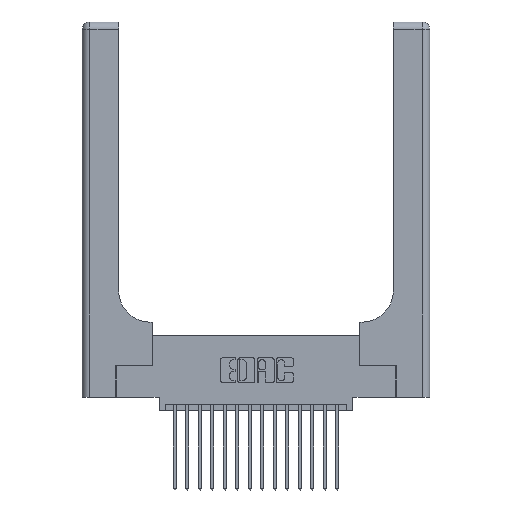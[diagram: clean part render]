
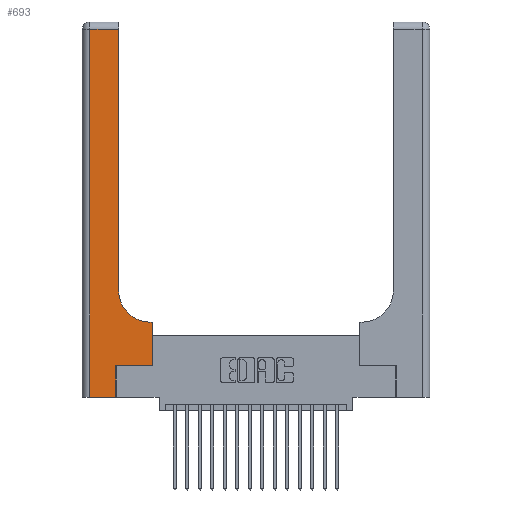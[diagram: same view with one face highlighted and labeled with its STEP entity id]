
A CAD part, top view. The second image highlights one B-rep face of the part: STEP entity #693.
In plain terms, the highlighted planar face has unit normal (0, 0, 1).
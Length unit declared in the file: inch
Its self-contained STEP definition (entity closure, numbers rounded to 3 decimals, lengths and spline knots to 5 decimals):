
#476 = PLANE ( 'NONE',  #8437 ) ;
#693 = ADVANCED_FACE ( 'NONE', ( #14383 ), #476, .F. ) ;
#715 = CARTESIAN_POINT ( 'NONE',  ( 0.5585, 0.25, 0.37 ) ) ;
#745 = CARTESIAN_POINT ( 'NONE',  ( 0.06, 2.94, 0.37 ) ) ;
#1092 = VERTEX_POINT ( 'NONE', #12189 ) ;
#1479 = DIRECTION ( 'NONE',  ( 1., 0., 0. ) ) ;
#2515 = ORIENTED_EDGE ( 'NONE', *, *, #7731, .T. ) ;
#2801 = VECTOR ( 'NONE', #18602, 39.37008 ) ;
#2877 = EDGE_CURVE ( 'NONE', #10043, #3869, #14999, .T. ) ;
#3142 = VERTEX_POINT ( 'NONE', #745 ) ;
#3202 = CARTESIAN_POINT ( 'NONE',  ( 0.269, 0., 0.37 ) ) ;
#3245 = ORIENTED_EDGE ( 'NONE', *, *, #9108, .T. ) ;
#3334 = CARTESIAN_POINT ( 'NONE',  ( 0.2915, 2.94, 0.37 ) ) ;
#3520 = ORIENTED_EDGE ( 'NONE', *, *, #2877, .T. ) ;
#3869 = VERTEX_POINT ( 'NONE', #10543 ) ;
#4021 = CARTESIAN_POINT ( 'NONE',  ( 0., 2.94, 0.37 ) ) ;
#4050 = CARTESIAN_POINT ( 'NONE',  ( 0., 3., 0.37 ) ) ;
#4329 = LINE ( 'NONE', #3202, #2801 ) ;
#4832 = DIRECTION ( 'NONE',  ( -1., 0., 0. ) ) ;
#4880 = CARTESIAN_POINT ( 'NONE',  ( 0., 0., 0.37 ) ) ;
#4991 = CARTESIAN_POINT ( 'NONE',  ( 0.2915, 0.6, 0.37 ) ) ;
#5069 = VERTEX_POINT ( 'NONE', #10572 ) ;
#5094 = CARTESIAN_POINT ( 'NONE',  ( 0.5415, 0.85, 0.37 ) ) ;
#6465 = VECTOR ( 'NONE', #4832, 39.37008 ) ;
#6475 = DIRECTION ( 'NONE',  ( 1., 0., 0. ) ) ;
#6684 = DIRECTION ( 'NONE',  ( 1., 0., 0. ) ) ;
#6845 = VERTEX_POINT ( 'NONE', #3334 ) ;
#7731 = EDGE_CURVE ( 'NONE', #12124, #10043, #16076, .T. ) ;
#7776 = ORIENTED_EDGE ( 'NONE', *, *, #17216, .T. ) ;
#8437 = AXIS2_PLACEMENT_3D ( 'NONE', #4050, #16220, #17780 ) ;
#8526 = EDGE_CURVE ( 'NONE', #5069, #12124, #15309, .T. ) ;
#8976 = ORIENTED_EDGE ( 'NONE', *, *, #17112, .T. ) ;
#9055 = VECTOR ( 'NONE', #6475, 39.37008 ) ;
#9108 = EDGE_CURVE ( 'NONE', #14019, #6845, #9429, .T. ) ;
#9429 = LINE ( 'NONE', #15978, #16958 ) ;
#9577 = CARTESIAN_POINT ( 'NONE',  ( 0.06, 3., 0.37 ) ) ;
#9667 = LINE ( 'NONE', #9577, #13173 ) ;
#10043 = VERTEX_POINT ( 'NONE', #12219 ) ;
#10425 = DIRECTION ( 'NONE',  ( -1., 0., 0. ) ) ;
#10543 = CARTESIAN_POINT ( 'NONE',  ( 0.5415, 0.6, 0.37 ) ) ;
#10572 = CARTESIAN_POINT ( 'NONE',  ( 0.269, 0.25, 0.37 ) ) ;
#11086 = DIRECTION ( 'NONE',  ( 0., -1., 0. ) ) ;
#11253 = CARTESIAN_POINT ( 'NONE',  ( 0.5585, 0.25, 0.37 ) ) ;
#11526 = VECTOR ( 'NONE', #10425, 39.37008 ) ;
#11546 = ORIENTED_EDGE ( 'NONE', *, *, #13515, .T. ) ;
#11577 = CARTESIAN_POINT ( 'NONE',  ( 0.2915, 0.85, 0.37 ) ) ;
#11626 = CIRCLE ( 'NONE', #13070, 0.25 ) ;
#11834 = EDGE_LOOP ( 'NONE', ( #3245, #11546, #12001, #8976, #13414, #13888, #2515, #3520, #7776 ) ) ;
#12001 = ORIENTED_EDGE ( 'NONE', *, *, #13152, .T. ) ;
#12124 = VERTEX_POINT ( 'NONE', #11253 ) ;
#12189 = CARTESIAN_POINT ( 'NONE',  ( 0.06, 0., 0.37 ) ) ;
#12219 = CARTESIAN_POINT ( 'NONE',  ( 0.5585, 0.6, 0.37 ) ) ;
#12281 = VERTEX_POINT ( 'NONE', #19182 ) ;
#12404 = CARTESIAN_POINT ( 'NONE',  ( 0.269, 0.25, 0.37 ) ) ;
#13030 = LINE ( 'NONE', #4880, #9055 ) ;
#13070 = AXIS2_PLACEMENT_3D ( 'NONE', #5094, #15761, #6684 ) ;
#13152 = EDGE_CURVE ( 'NONE', #3142, #1092, #9667, .T. ) ;
#13173 = VECTOR ( 'NONE', #11086, 39.37008 ) ;
#13234 = DIRECTION ( 'NONE',  ( 0., 1., 0. ) ) ;
#13414 = ORIENTED_EDGE ( 'NONE', *, *, #18246, .T. ) ;
#13515 = EDGE_CURVE ( 'NONE', #6845, #3142, #15507, .T. ) ;
#13888 = ORIENTED_EDGE ( 'NONE', *, *, #8526, .T. ) ;
#14019 = VERTEX_POINT ( 'NONE', #11577 ) ;
#14383 = FACE_OUTER_BOUND ( 'NONE', #11834, .T. ) ;
#14844 = VECTOR ( 'NONE', #1479, 39.37008 ) ;
#14999 = LINE ( 'NONE', #4991, #6465 ) ;
#15309 = LINE ( 'NONE', #12404, #14844 ) ;
#15507 = LINE ( 'NONE', #4021, #11526 ) ;
#15761 = DIRECTION ( 'NONE',  ( 0., 0., -1. ) ) ;
#15978 = CARTESIAN_POINT ( 'NONE',  ( 0.2915, 3., 0.37 ) ) ;
#16076 = LINE ( 'NONE', #715, #19622 ) ;
#16220 = DIRECTION ( 'NONE',  ( 0., 0., -1. ) ) ;
#16958 = VECTOR ( 'NONE', #17511, 39.37008 ) ;
#17112 = EDGE_CURVE ( 'NONE', #1092, #12281, #13030, .T. ) ;
#17216 = EDGE_CURVE ( 'NONE', #3869, #14019, #11626, .T. ) ;
#17511 = DIRECTION ( 'NONE',  ( 0., 1., 0. ) ) ;
#17780 = DIRECTION ( 'NONE',  ( -1., 0., 0. ) ) ;
#18246 = EDGE_CURVE ( 'NONE', #12281, #5069, #4329, .T. ) ;
#18602 = DIRECTION ( 'NONE',  ( 0., 1., 0. ) ) ;
#19182 = CARTESIAN_POINT ( 'NONE',  ( 0.269, 0., 0.37 ) ) ;
#19622 = VECTOR ( 'NONE', #13234, 39.37008 ) ;
